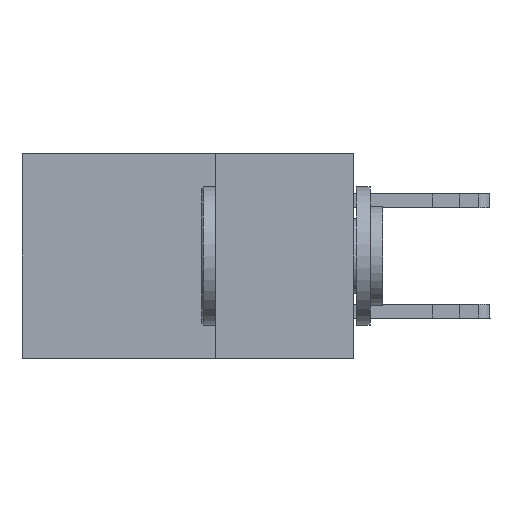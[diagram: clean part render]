
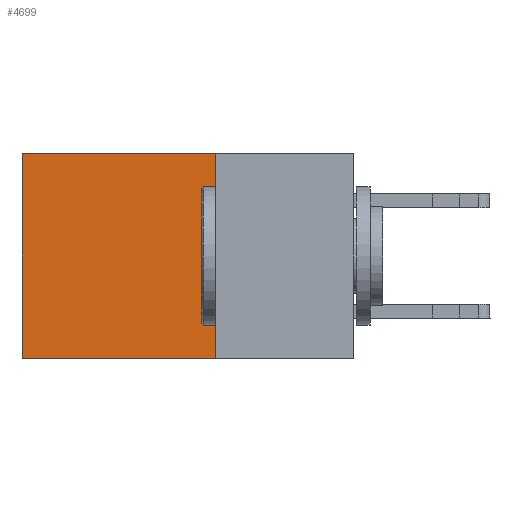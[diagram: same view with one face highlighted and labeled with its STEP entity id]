
A CAD part, left-side view. The second image highlights one B-rep face of the part: STEP entity #4699.
In plain terms, the highlighted planar face has unit normal (-1, 0, 0).
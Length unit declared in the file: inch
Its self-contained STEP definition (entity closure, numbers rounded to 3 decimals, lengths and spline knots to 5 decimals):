
#281 = VERTEX_POINT ( 'NONE', #301 ) ;
#301 = CARTESIAN_POINT ( 'NONE',  ( 0.2875, 0.25, 0. ) ) ;
#1168 = EDGE_CURVE ( 'NONE', #281, #14530, #11560, .T. ) ;
#1883 = ORIENTED_EDGE ( 'NONE', *, *, #1168, .F. ) ;
#3486 = EDGE_CURVE ( 'NONE', #281, #15884, #21794, .T. ) ;
#3656 = CARTESIAN_POINT ( 'NONE',  ( 0.2875, 0.25, 0. ) ) ;
#3715 = CARTESIAN_POINT ( 'NONE',  ( 0.2875, 0.25, 0. ) ) ;
#4306 = CARTESIAN_POINT ( 'NONE',  ( 0.2875, 0.25, -0.37 ) ) ;
#4699 = ADVANCED_FACE ( 'NONE', ( #6142 ), #17387, .F. ) ;
#5504 = EDGE_CURVE ( 'NONE', #14530, #10048, #9531, .T. ) ;
#5562 = VECTOR ( 'NONE', #14604, 39.37008 ) ;
#5626 = CARTESIAN_POINT ( 'NONE',  ( 0.2875, 0.25, 0. ) ) ;
#6142 = FACE_OUTER_BOUND ( 'NONE', #6698, .T. ) ;
#6698 = EDGE_LOOP ( 'NONE', ( #11408, #19300, #1883, #6865 ) ) ;
#6865 = ORIENTED_EDGE ( 'NONE', *, *, #3486, .T. ) ;
#6994 = VECTOR ( 'NONE', #10084, 39.37008 ) ;
#7082 = DIRECTION ( 'NONE',  ( 1., 0., 0. ) ) ;
#8160 = CARTESIAN_POINT ( 'NONE',  ( 0.2875, 0.25, -0.37 ) ) ;
#8868 = DIRECTION ( 'NONE',  ( 0., 1., 0. ) ) ;
#8963 = AXIS2_PLACEMENT_3D ( 'NONE', #3656, #7082, #19159 ) ;
#9531 = LINE ( 'NONE', #4306, #5562 ) ;
#9952 = CARTESIAN_POINT ( 'NONE',  ( 0.2875, 0.6, 0. ) ) ;
#10048 = VERTEX_POINT ( 'NONE', #21995 ) ;
#10084 = DIRECTION ( 'NONE',  ( 0., 0., -1. ) ) ;
#11395 = CARTESIAN_POINT ( 'NONE',  ( 0.2875, 0.6, 0. ) ) ;
#11408 = ORIENTED_EDGE ( 'NONE', *, *, #18679, .T. ) ;
#11560 = LINE ( 'NONE', #5626, #6994 ) ;
#12094 = VECTOR ( 'NONE', #8868, 39.37008 ) ;
#12579 = VECTOR ( 'NONE', #18273, 39.37008 ) ;
#13118 = LINE ( 'NONE', #11395, #12579 ) ;
#14530 = VERTEX_POINT ( 'NONE', #8160 ) ;
#14604 = DIRECTION ( 'NONE',  ( 0., 1., 0. ) ) ;
#15884 = VERTEX_POINT ( 'NONE', #9952 ) ;
#17387 = PLANE ( 'NONE',  #8963 ) ;
#18273 = DIRECTION ( 'NONE',  ( 0., 0., -1. ) ) ;
#18679 = EDGE_CURVE ( 'NONE', #15884, #10048, #13118, .T. ) ;
#19159 = DIRECTION ( 'NONE',  ( 0., 0., -1. ) ) ;
#19300 = ORIENTED_EDGE ( 'NONE', *, *, #5504, .F. ) ;
#21794 = LINE ( 'NONE', #3715, #12094 ) ;
#21995 = CARTESIAN_POINT ( 'NONE',  ( 0.2875, 0.6, -0.37 ) ) ;
